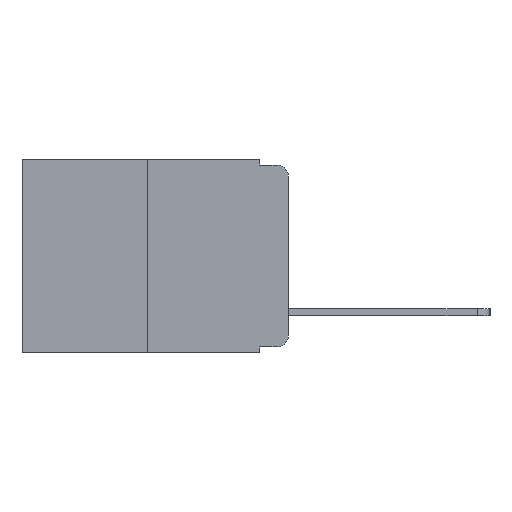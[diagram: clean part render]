
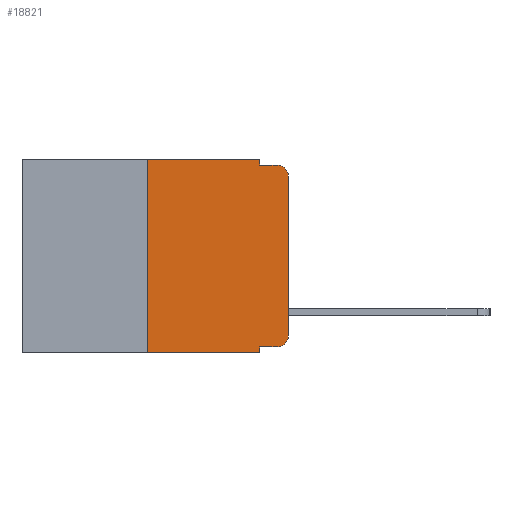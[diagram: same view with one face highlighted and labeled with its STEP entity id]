
A CAD part, left-side view. The second image highlights one B-rep face of the part: STEP entity #18821.
In plain terms, the highlighted planar face has unit normal (-1, 0, 0).
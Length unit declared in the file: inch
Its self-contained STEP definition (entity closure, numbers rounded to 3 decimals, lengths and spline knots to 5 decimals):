
#21 = EDGE_CURVE ( 'NONE', #18107, #8475, #13289, .T. ) ;
#137 = VERTEX_POINT ( 'NONE', #12225 ) ;
#693 = PLANE ( 'NONE',  #855 ) ;
#855 = AXIS2_PLACEMENT_3D ( 'NONE', #11939, #2359, #13517 ) ;
#1179 = EDGE_CURVE ( 'NONE', #17161, #18107, #4766, .T. ) ;
#1289 = DIRECTION ( 'NONE',  ( 0., 0., -1. ) ) ;
#1382 = DIRECTION ( 'NONE',  ( 0., -1., 0. ) ) ;
#1461 = EDGE_CURVE ( 'NONE', #137, #5079, #7284, .T. ) ;
#2280 = EDGE_CURVE ( 'NONE', #17161, #5079, #13457, .T. ) ;
#2359 = DIRECTION ( 'NONE',  ( 1., 0., 0. ) ) ;
#2874 = CARTESIAN_POINT ( 'NONE',  ( 0., 0.051, -0.343 ) ) ;
#2933 = AXIS2_PLACEMENT_3D ( 'NONE', #15260, #14919, #14832 ) ;
#3147 = ORIENTED_EDGE ( 'NONE', *, *, #2280, .F. ) ;
#3399 = EDGE_CURVE ( 'NONE', #137, #13046, #14860, .T. ) ;
#3505 = CARTESIAN_POINT ( 'NONE',  ( 0., 0.051, -0.01 ) ) ;
#3573 = DIRECTION ( 'NONE',  ( 0., -1., 0. ) ) ;
#3966 = CARTESIAN_POINT ( 'NONE',  ( 0., 0.051, -0.01 ) ) ;
#4766 = LINE ( 'NONE', #9401, #12757 ) ;
#4871 = DIRECTION ( 'NONE',  ( 0., 0., 1. ) ) ;
#5017 = CARTESIAN_POINT ( 'NONE',  ( 0., 0.473, -0.343 ) ) ;
#5079 = VERTEX_POINT ( 'NONE', #2874 ) ;
#5511 = EDGE_CURVE ( 'NONE', #10843, #7334, #13088, .T. ) ;
#5777 = ORIENTED_EDGE ( 'NONE', *, *, #21, .T. ) ;
#5798 = DIRECTION ( 'NONE',  ( -1., 0., 0. ) ) ;
#6043 = CARTESIAN_POINT ( 'NONE',  ( 0., 0.051, 0. ) ) ;
#6380 = ORIENTED_EDGE ( 'NONE', *, *, #1461, .T. ) ;
#6546 = VERTEX_POINT ( 'NONE', #14838 ) ;
#6598 = EDGE_CURVE ( 'NONE', #7334, #6546, #7755, .T. ) ;
#6705 = VECTOR ( 'NONE', #1382, 39.37008 ) ;
#6720 = CARTESIAN_POINT ( 'NONE',  ( 0., 0.051, 0. ) ) ;
#6818 = CARTESIAN_POINT ( 'NONE',  ( 0., 0.02, -0.333 ) ) ;
#6827 = CARTESIAN_POINT ( 'NONE',  ( 0., 0., -0.03 ) ) ;
#7192 = VERTEX_POINT ( 'NONE', #6827 ) ;
#7284 = LINE ( 'NONE', #5017, #11014 ) ;
#7334 = VERTEX_POINT ( 'NONE', #3966 ) ;
#7625 = ORIENTED_EDGE ( 'NONE', *, *, #7646, .T. ) ;
#7646 = EDGE_CURVE ( 'NONE', #7192, #6546, #7959, .T. ) ;
#7755 = LINE ( 'NONE', #3505, #19139 ) ;
#7959 = CIRCLE ( 'NONE', #2933, 0.02 ) ;
#8106 = ORIENTED_EDGE ( 'NONE', *, *, #6598, .F. ) ;
#8110 = DIRECTION ( 'NONE',  ( 0., -1., 0. ) ) ;
#8475 = VERTEX_POINT ( 'NONE', #12825 ) ;
#8668 = EDGE_LOOP ( 'NONE', ( #13073, #7625, #8106, #19470, #9599, #19732, #6380, #3147, #18046, #5777 ) ) ;
#8708 = EDGE_CURVE ( 'NONE', #8475, #7192, #13183, .T. ) ;
#8951 = VECTOR ( 'NONE', #4871, 39.37008 ) ;
#9115 = EDGE_CURVE ( 'NONE', #13046, #10843, #10934, .T. ) ;
#9349 = VECTOR ( 'NONE', #1289, 39.37008 ) ;
#9401 = CARTESIAN_POINT ( 'NONE',  ( 0., 0.051, -0.333 ) ) ;
#9442 = CARTESIAN_POINT ( 'NONE',  ( 0., 0.02, -0.313 ) ) ;
#9599 = ORIENTED_EDGE ( 'NONE', *, *, #9115, .F. ) ;
#9643 = CARTESIAN_POINT ( 'NONE',  ( 0., 0.473, 0. ) ) ;
#10289 = CARTESIAN_POINT ( 'NONE',  ( 0., 0.25, 0. ) ) ;
#10352 = CARTESIAN_POINT ( 'NONE',  ( 0., 0.25, 0. ) ) ;
#10843 = VERTEX_POINT ( 'NONE', #6043 ) ;
#10934 = LINE ( 'NONE', #9643, #6705 ) ;
#10993 = DIRECTION ( 'NONE',  ( 0., -1., 0. ) ) ;
#11014 = VECTOR ( 'NONE', #10993, 39.37008 ) ;
#11939 = CARTESIAN_POINT ( 'NONE',  ( 0., 0.473, 0. ) ) ;
#12223 = CARTESIAN_POINT ( 'NONE',  ( 0., 0., 0. ) ) ;
#12225 = CARTESIAN_POINT ( 'NONE',  ( 0., 0.25, -0.343 ) ) ;
#12350 = DIRECTION ( 'NONE',  ( 0., 0., 1. ) ) ;
#12427 = AXIS2_PLACEMENT_3D ( 'NONE', #9442, #5798, #15874 ) ;
#12757 = VECTOR ( 'NONE', #8110, 39.37008 ) ;
#12825 = CARTESIAN_POINT ( 'NONE',  ( 0., 0., -0.313 ) ) ;
#13046 = VERTEX_POINT ( 'NONE', #10289 ) ;
#13073 = ORIENTED_EDGE ( 'NONE', *, *, #8708, .T. ) ;
#13088 = LINE ( 'NONE', #15290, #9349 ) ;
#13183 = LINE ( 'NONE', #12223, #8951 ) ;
#13289 = CIRCLE ( 'NONE', #12427, 0.02 ) ;
#13442 = VECTOR ( 'NONE', #12350, 39.37008 ) ;
#13457 = LINE ( 'NONE', #6720, #16512 ) ;
#13517 = DIRECTION ( 'NONE',  ( 0., 0., -1. ) ) ;
#14552 = CARTESIAN_POINT ( 'NONE',  ( 0., 0.051, -0.333 ) ) ;
#14832 = DIRECTION ( 'NONE',  ( 0., 0., -1. ) ) ;
#14838 = CARTESIAN_POINT ( 'NONE',  ( 0., 0.02, -0.01 ) ) ;
#14860 = LINE ( 'NONE', #10352, #13442 ) ;
#14919 = DIRECTION ( 'NONE',  ( -1., 0., 0. ) ) ;
#15260 = CARTESIAN_POINT ( 'NONE',  ( 0., 0.02, -0.03 ) ) ;
#15290 = CARTESIAN_POINT ( 'NONE',  ( 0., 0.051, 0. ) ) ;
#15874 = DIRECTION ( 'NONE',  ( 0., 0., -1. ) ) ;
#16512 = VECTOR ( 'NONE', #16919, 39.37008 ) ;
#16919 = DIRECTION ( 'NONE',  ( 0., 0., -1. ) ) ;
#17161 = VERTEX_POINT ( 'NONE', #14552 ) ;
#17853 = FACE_OUTER_BOUND ( 'NONE', #8668, .T. ) ;
#18046 = ORIENTED_EDGE ( 'NONE', *, *, #1179, .T. ) ;
#18107 = VERTEX_POINT ( 'NONE', #6818 ) ;
#18821 = ADVANCED_FACE ( 'NONE', ( #17853 ), #693, .F. ) ;
#19139 = VECTOR ( 'NONE', #3573, 39.37008 ) ;
#19470 = ORIENTED_EDGE ( 'NONE', *, *, #5511, .F. ) ;
#19732 = ORIENTED_EDGE ( 'NONE', *, *, #3399, .F. ) ;
